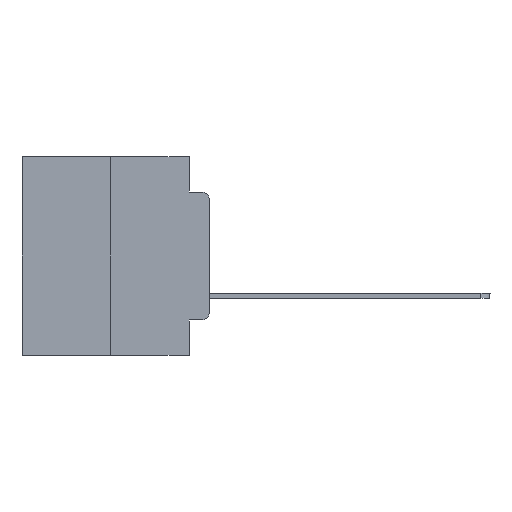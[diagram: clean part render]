
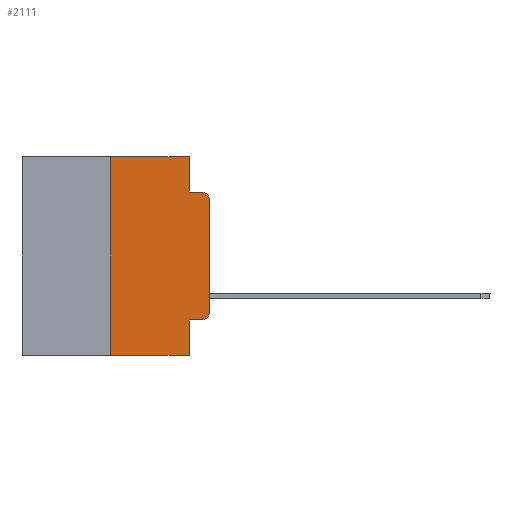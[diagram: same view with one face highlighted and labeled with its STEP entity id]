
A CAD part, left-side view. The second image highlights one B-rep face of the part: STEP entity #2111.
In plain terms, the highlighted planar face has unit normal (-1, 0, 0).
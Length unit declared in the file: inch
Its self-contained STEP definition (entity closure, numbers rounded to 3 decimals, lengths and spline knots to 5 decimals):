
#541 = ORIENTED_EDGE ( 'NONE', *, *, #19565, .T. ) ;
#1014 = DIRECTION ( 'NONE',  ( 0., 0., 1. ) ) ;
#1398 = LINE ( 'NONE', #3690, #12554 ) ;
#1780 = LINE ( 'NONE', #25884, #16943 ) ;
#1983 = ORIENTED_EDGE ( 'NONE', *, *, #5942, .T. ) ;
#2111 = ADVANCED_FACE ( 'NONE', ( #12168 ), #8255, .F. ) ;
#2293 = LINE ( 'NONE', #3886, #12268 ) ;
#2525 = DIRECTION ( 'NONE',  ( -1., 0., 0. ) ) ;
#3090 = CIRCLE ( 'NONE', #19129, 0.02 ) ;
#3690 = CARTESIAN_POINT ( 'NONE',  ( 0., 0.473, -0.5 ) ) ;
#3886 = CARTESIAN_POINT ( 'NONE',  ( 0., 0.051, 0. ) ) ;
#5108 = VECTOR ( 'NONE', #13133, 39.37008 ) ;
#5120 = CARTESIAN_POINT ( 'NONE',  ( 0., 0.25, 0. ) ) ;
#5942 = EDGE_CURVE ( 'NONE', #7849, #21571, #24542, .T. ) ;
#5999 = CARTESIAN_POINT ( 'NONE',  ( 0., 0.25, 0. ) ) ;
#6073 = CARTESIAN_POINT ( 'NONE',  ( 0., 0.051, -0.0885 ) ) ;
#6670 = ORIENTED_EDGE ( 'NONE', *, *, #11329, .F. ) ;
#7180 = ORIENTED_EDGE ( 'NONE', *, *, #7842, .F. ) ;
#7327 = EDGE_LOOP ( 'NONE', ( #1983, #9122, #10545, #11362, #6670, #7180, #27489, #8839, #20321, #541 ) ) ;
#7337 = LINE ( 'NONE', #13962, #14985 ) ;
#7806 = CIRCLE ( 'NONE', #27522, 0.02 ) ;
#7842 = EDGE_CURVE ( 'NONE', #16398, #27743, #27796, .T. ) ;
#7849 = VERTEX_POINT ( 'NONE', #21337 ) ;
#7947 = CARTESIAN_POINT ( 'NONE',  ( 0., 0.051, -0.5 ) ) ;
#7972 = CARTESIAN_POINT ( 'NONE',  ( 0., 0.051, -0.4115 ) ) ;
#8255 = PLANE ( 'NONE',  #14062 ) ;
#8839 = ORIENTED_EDGE ( 'NONE', *, *, #18803, .F. ) ;
#9122 = ORIENTED_EDGE ( 'NONE', *, *, #10773, .T. ) ;
#9826 = EDGE_CURVE ( 'NONE', #19664, #20645, #1780, .T. ) ;
#10308 = EDGE_CURVE ( 'NONE', #28284, #24412, #12102, .T. ) ;
#10545 = ORIENTED_EDGE ( 'NONE', *, *, #10308, .F. ) ;
#10773 = EDGE_CURVE ( 'NONE', #21571, #24412, #7806, .T. ) ;
#11231 = DIRECTION ( 'NONE',  ( 0., 0., -1. ) ) ;
#11329 = EDGE_CURVE ( 'NONE', #27743, #25368, #19567, .T. ) ;
#11362 = ORIENTED_EDGE ( 'NONE', *, *, #18604, .F. ) ;
#12100 = CARTESIAN_POINT ( 'NONE',  ( 0., 0.02, -0.0885 ) ) ;
#12102 = LINE ( 'NONE', #16562, #13777 ) ;
#12168 = FACE_OUTER_BOUND ( 'NONE', #7327, .T. ) ;
#12268 = VECTOR ( 'NONE', #19367, 39.37008 ) ;
#12528 = DIRECTION ( 'NONE',  ( 0., -1., 0. ) ) ;
#12554 = VECTOR ( 'NONE', #16621, 39.37008 ) ;
#12740 = DIRECTION ( 'NONE',  ( 0., 0., -1. ) ) ;
#13133 = DIRECTION ( 'NONE',  ( 0., -1., 0. ) ) ;
#13596 = DIRECTION ( 'NONE',  ( 0., 0., -1. ) ) ;
#13777 = VECTOR ( 'NONE', #12528, 39.37008 ) ;
#13962 = CARTESIAN_POINT ( 'NONE',  ( 0., 0.051, 0. ) ) ;
#14062 = AXIS2_PLACEMENT_3D ( 'NONE', #23188, #18607, #12740 ) ;
#14208 = VECTOR ( 'NONE', #25646, 39.37008 ) ;
#14630 = CARTESIAN_POINT ( 'NONE',  ( 0., 0.051, 0. ) ) ;
#14985 = VECTOR ( 'NONE', #11231, 39.37008 ) ;
#16185 = DIRECTION ( 'NONE',  ( 0., 0., -1. ) ) ;
#16398 = VERTEX_POINT ( 'NONE', #19973 ) ;
#16562 = CARTESIAN_POINT ( 'NONE',  ( 0., 0.051, -0.0885 ) ) ;
#16621 = DIRECTION ( 'NONE',  ( 0., -1., 0. ) ) ;
#16943 = VECTOR ( 'NONE', #23155, 39.37008 ) ;
#18312 = CARTESIAN_POINT ( 'NONE',  ( 0., 0.02, -0.3915 ) ) ;
#18604 = EDGE_CURVE ( 'NONE', #25368, #28284, #7337, .T. ) ;
#18607 = DIRECTION ( 'NONE',  ( 1., 0., 0. ) ) ;
#18803 = EDGE_CURVE ( 'NONE', #19664, #23878, #2293, .T. ) ;
#19129 = AXIS2_PLACEMENT_3D ( 'NONE', #18312, #27069, #16185 ) ;
#19367 = DIRECTION ( 'NONE',  ( 0., 0., -1. ) ) ;
#19565 = EDGE_CURVE ( 'NONE', #20645, #7849, #3090, .T. ) ;
#19567 = LINE ( 'NONE', #28325, #5108 ) ;
#19664 = VERTEX_POINT ( 'NONE', #7972 ) ;
#19973 = CARTESIAN_POINT ( 'NONE',  ( 0., 0.25, -0.5 ) ) ;
#19977 = CARTESIAN_POINT ( 'NONE',  ( 0., 0., -0.1085 ) ) ;
#20321 = ORIENTED_EDGE ( 'NONE', *, *, #9826, .T. ) ;
#20482 = CARTESIAN_POINT ( 'NONE',  ( 0., 0.02, -0.4115 ) ) ;
#20645 = VERTEX_POINT ( 'NONE', #20482 ) ;
#20670 = CARTESIAN_POINT ( 'NONE',  ( 0., 0., 0. ) ) ;
#21337 = CARTESIAN_POINT ( 'NONE',  ( 0., 0., -0.3915 ) ) ;
#21571 = VERTEX_POINT ( 'NONE', #19977 ) ;
#22918 = VECTOR ( 'NONE', #1014, 39.37008 ) ;
#23155 = DIRECTION ( 'NONE',  ( 0., -1., 0. ) ) ;
#23188 = CARTESIAN_POINT ( 'NONE',  ( 0., 0.473, 0. ) ) ;
#23483 = EDGE_CURVE ( 'NONE', #16398, #23878, #1398, .T. ) ;
#23878 = VERTEX_POINT ( 'NONE', #7947 ) ;
#24412 = VERTEX_POINT ( 'NONE', #12100 ) ;
#24472 = CARTESIAN_POINT ( 'NONE',  ( 0., 0.02, -0.1085 ) ) ;
#24542 = LINE ( 'NONE', #20670, #22918 ) ;
#25368 = VERTEX_POINT ( 'NONE', #14630 ) ;
#25646 = DIRECTION ( 'NONE',  ( 0., 0., 1. ) ) ;
#25884 = CARTESIAN_POINT ( 'NONE',  ( 0., 0.051, -0.4115 ) ) ;
#27069 = DIRECTION ( 'NONE',  ( -1., 0., 0. ) ) ;
#27489 = ORIENTED_EDGE ( 'NONE', *, *, #23483, .T. ) ;
#27522 = AXIS2_PLACEMENT_3D ( 'NONE', #24472, #2525, #13596 ) ;
#27743 = VERTEX_POINT ( 'NONE', #5120 ) ;
#27796 = LINE ( 'NONE', #5999, #14208 ) ;
#28284 = VERTEX_POINT ( 'NONE', #6073 ) ;
#28325 = CARTESIAN_POINT ( 'NONE',  ( 0., 0.473, 0. ) ) ;
